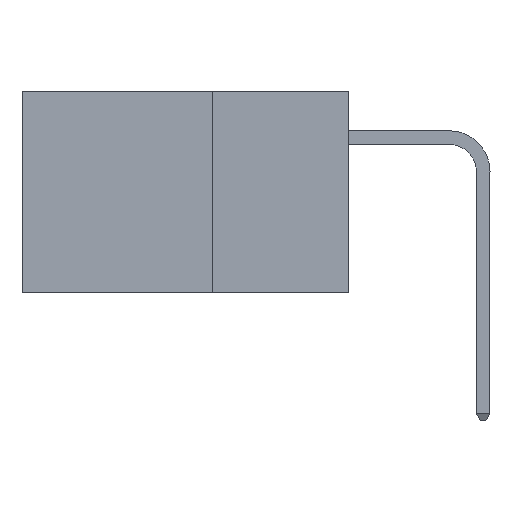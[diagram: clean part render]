
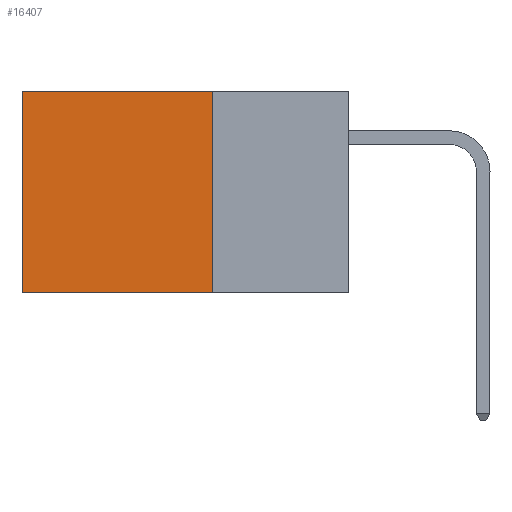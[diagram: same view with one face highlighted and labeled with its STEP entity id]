
A CAD part, left-side view. The second image highlights one B-rep face of the part: STEP entity #16407.
In plain terms, the highlighted planar face has unit normal (-1, 0, 0).
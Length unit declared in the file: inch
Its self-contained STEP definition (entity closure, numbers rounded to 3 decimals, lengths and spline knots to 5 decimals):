
#405 = CARTESIAN_POINT ( 'NONE',  ( 0.2875, 0.25, -0.37 ) ) ;
#551 = EDGE_CURVE ( 'NONE', #14227, #21285, #624, .T. ) ;
#624 = LINE ( 'NONE', #12672, #13056 ) ;
#1780 = FACE_OUTER_BOUND ( 'NONE', #3057, .T. ) ;
#3057 = EDGE_LOOP ( 'NONE', ( #4433, #16102, #9845, #3083 ) ) ;
#3083 = ORIENTED_EDGE ( 'NONE', *, *, #551, .T. ) ;
#4433 = ORIENTED_EDGE ( 'NONE', *, *, #10777, .T. ) ;
#5461 = VECTOR ( 'NONE', #10959, 39.37008 ) ;
#5779 = PLANE ( 'NONE',  #12988 ) ;
#7242 = CARTESIAN_POINT ( 'NONE',  ( 0.2875, 0.25, -0.37 ) ) ;
#7479 = DIRECTION ( 'NONE',  ( 0., 0., -1. ) ) ;
#9283 = CARTESIAN_POINT ( 'NONE',  ( 0.2875, 0.6, 0. ) ) ;
#9845 = ORIENTED_EDGE ( 'NONE', *, *, #13301, .F. ) ;
#9955 = LINE ( 'NONE', #9283, #5461 ) ;
#10777 = EDGE_CURVE ( 'NONE', #21285, #16211, #9955, .T. ) ;
#10959 = DIRECTION ( 'NONE',  ( 0., 0., -1. ) ) ;
#11636 = CARTESIAN_POINT ( 'NONE',  ( 0.2875, 0.25, 0. ) ) ;
#11946 = CARTESIAN_POINT ( 'NONE',  ( 0.2875, 0.6, 0. ) ) ;
#12174 = EDGE_CURVE ( 'NONE', #20255, #16211, #16955, .T. ) ;
#12501 = VECTOR ( 'NONE', #17303, 39.37008 ) ;
#12672 = CARTESIAN_POINT ( 'NONE',  ( 0.2875, 0.25, 0. ) ) ;
#12708 = LINE ( 'NONE', #14522, #20504 ) ;
#12988 = AXIS2_PLACEMENT_3D ( 'NONE', #15825, #17490, #7479 ) ;
#13056 = VECTOR ( 'NONE', #14369, 39.37008 ) ;
#13301 = EDGE_CURVE ( 'NONE', #14227, #20255, #12708, .T. ) ;
#14227 = VERTEX_POINT ( 'NONE', #11636 ) ;
#14369 = DIRECTION ( 'NONE',  ( 0., 1., 0. ) ) ;
#14522 = CARTESIAN_POINT ( 'NONE',  ( 0.2875, 0.25, 0. ) ) ;
#15825 = CARTESIAN_POINT ( 'NONE',  ( 0.2875, 0.25, 0. ) ) ;
#16102 = ORIENTED_EDGE ( 'NONE', *, *, #12174, .F. ) ;
#16196 = DIRECTION ( 'NONE',  ( 0., 0., -1. ) ) ;
#16211 = VERTEX_POINT ( 'NONE', #17007 ) ;
#16407 = ADVANCED_FACE ( 'NONE', ( #1780 ), #5779, .F. ) ;
#16955 = LINE ( 'NONE', #405, #12501 ) ;
#17007 = CARTESIAN_POINT ( 'NONE',  ( 0.2875, 0.6, -0.37 ) ) ;
#17303 = DIRECTION ( 'NONE',  ( 0., 1., 0. ) ) ;
#17490 = DIRECTION ( 'NONE',  ( 1., 0., 0. ) ) ;
#20255 = VERTEX_POINT ( 'NONE', #7242 ) ;
#20504 = VECTOR ( 'NONE', #16196, 39.37008 ) ;
#21285 = VERTEX_POINT ( 'NONE', #11946 ) ;
